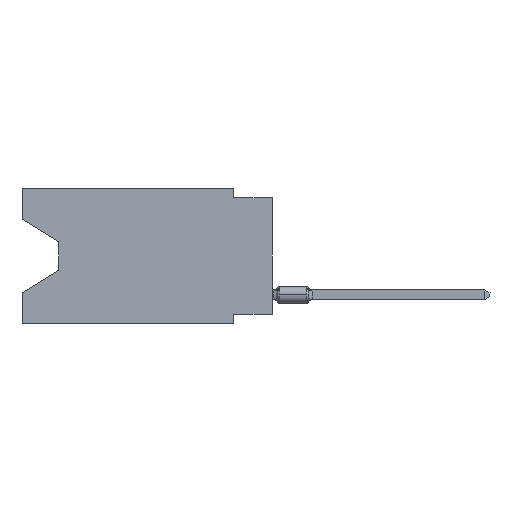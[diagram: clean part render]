
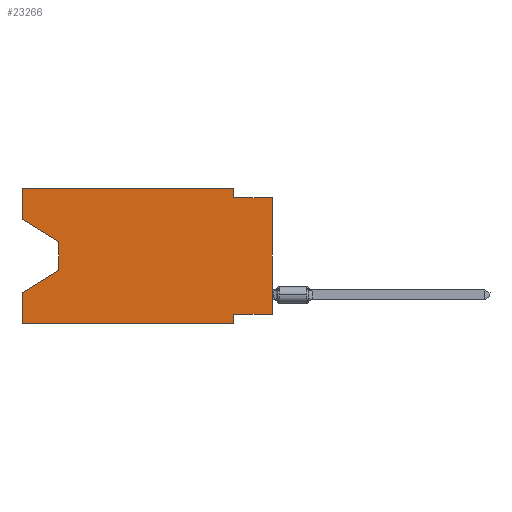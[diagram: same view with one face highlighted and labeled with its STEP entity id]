
A CAD part, left-side view. The second image highlights one B-rep face of the part: STEP entity #23266.
In plain terms, the highlighted planar face has unit normal (-1, 0, 0).
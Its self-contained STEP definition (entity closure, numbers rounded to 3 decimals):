
#442 = EDGE_CURVE ( 'NONE', #22999, #3769, #12356, .T. ) ;
#644 = DIRECTION ( 'NONE',  ( 0., -0.855, -0.519 ) ) ;
#653 = VERTEX_POINT ( 'NONE', #32767 ) ;
#2056 = DIRECTION ( 'NONE',  ( 0., 0., -1. ) ) ;
#2120 = LINE ( 'NONE', #27489, #5346 ) ;
#2389 = VECTOR ( 'NONE', #644, 1000. ) ;
#2647 = CARTESIAN_POINT ( 'NONE',  ( 0., 2.54, 0. ) ) ;
#2671 = EDGE_CURVE ( 'NONE', #15702, #17111, #13819, .T. ) ;
#3279 = DIRECTION ( 'NONE',  ( 0., -1., 0. ) ) ;
#3314 = LINE ( 'NONE', #16324, #17776 ) ;
#3705 = CARTESIAN_POINT ( 'NONE',  ( 0., 16.383, -6.852 ) ) ;
#3769 = VERTEX_POINT ( 'NONE', #3705 ) ;
#4119 = EDGE_CURVE ( 'NONE', #17111, #22999, #9005, .T. ) ;
#5346 = VECTOR ( 'NONE', #17646, 1000. ) ;
#5392 = DIRECTION ( 'NONE',  ( 0., -1., 0. ) ) ;
#5425 = ORIENTED_EDGE ( 'NONE', *, *, #5954, .T. ) ;
#5474 = CARTESIAN_POINT ( 'NONE',  ( 0., 16.383, 0. ) ) ;
#5954 = EDGE_CURVE ( 'NONE', #28334, #21134, #17801, .T. ) ;
#6075 = LINE ( 'NONE', #13913, #18885 ) ;
#6203 = CARTESIAN_POINT ( 'NONE',  ( 0., 13.97, -3.505 ) ) ;
#6635 = ORIENTED_EDGE ( 'NONE', *, *, #13064, .F. ) ;
#7276 = DIRECTION ( 'NONE',  ( 0., 1., 0. ) ) ;
#8796 = VERTEX_POINT ( 'NONE', #28716 ) ;
#9005 = LINE ( 'NONE', #11507, #21116 ) ;
#9385 = VECTOR ( 'NONE', #5392, 1000. ) ;
#9765 = DIRECTION ( 'NONE',  ( 0., -1., 0. ) ) ;
#9788 = ORIENTED_EDGE ( 'NONE', *, *, #12281, .F. ) ;
#9918 = LINE ( 'NONE', #14455, #26642 ) ;
#11176 = CARTESIAN_POINT ( 'NONE',  ( 0., 0., -0.635 ) ) ;
#11317 = DIRECTION ( 'NONE',  ( 0., 0., -1. ) ) ;
#11507 = CARTESIAN_POINT ( 'NONE',  ( 0., 13.97, -3.505 ) ) ;
#12281 = EDGE_CURVE ( 'NONE', #29507, #12724, #3314, .T. ) ;
#12282 = CARTESIAN_POINT ( 'NONE',  ( 0., 2.54, -8.89 ) ) ;
#12356 = LINE ( 'NONE', #27379, #27001 ) ;
#12519 = VECTOR ( 'NONE', #14032, 1000. ) ;
#12667 = ORIENTED_EDGE ( 'NONE', *, *, #13554, .T. ) ;
#12724 = VERTEX_POINT ( 'NONE', #24295 ) ;
#13064 = EDGE_CURVE ( 'NONE', #28334, #3769, #6075, .T. ) ;
#13280 = AXIS2_PLACEMENT_3D ( 'NONE', #20258, #15070, #2056 ) ;
#13554 = EDGE_CURVE ( 'NONE', #8796, #32348, #27857, .T. ) ;
#13819 = LINE ( 'NONE', #23676, #2389 ) ;
#13913 = CARTESIAN_POINT ( 'NONE',  ( 0., 16.383, 0. ) ) ;
#14032 = DIRECTION ( 'NONE',  ( 0., 0., 1. ) ) ;
#14408 = ORIENTED_EDGE ( 'NONE', *, *, #29899, .F. ) ;
#14455 = CARTESIAN_POINT ( 'NONE',  ( 0., 0., -8.255 ) ) ;
#14569 = FACE_OUTER_BOUND ( 'NONE', #31583, .T. ) ;
#14608 = DIRECTION ( 'NONE',  ( 0., 0., -1. ) ) ;
#14662 = CARTESIAN_POINT ( 'NONE',  ( 0., 16.383, 0. ) ) ;
#15070 = DIRECTION ( 'NONE',  ( 1., 0., 0. ) ) ;
#15702 = VERTEX_POINT ( 'NONE', #22621 ) ;
#16131 = ORIENTED_EDGE ( 'NONE', *, *, #31618, .F. ) ;
#16324 = CARTESIAN_POINT ( 'NONE',  ( 0., 2.54, 0. ) ) ;
#17111 = VERTEX_POINT ( 'NONE', #6203 ) ;
#17641 = VERTEX_POINT ( 'NONE', #14662 ) ;
#17646 = DIRECTION ( 'NONE',  ( 0., 0., 1. ) ) ;
#17701 = ORIENTED_EDGE ( 'NONE', *, *, #18612, .F. ) ;
#17754 = EDGE_CURVE ( 'NONE', #12724, #32348, #20912, .T. ) ;
#17776 = VECTOR ( 'NONE', #11317, 1000. ) ;
#17801 = LINE ( 'NONE', #32835, #26101 ) ;
#18319 = LINE ( 'NONE', #5474, #30921 ) ;
#18461 = ORIENTED_EDGE ( 'NONE', *, *, #2671, .T. ) ;
#18612 = EDGE_CURVE ( 'NONE', #653, #21134, #27471, .T. ) ;
#18692 = ORIENTED_EDGE ( 'NONE', *, *, #442, .T. ) ;
#18885 = VECTOR ( 'NONE', #20946, 1000. ) ;
#20258 = CARTESIAN_POINT ( 'NONE',  ( 0., 16.383, 0. ) ) ;
#20323 = ORIENTED_EDGE ( 'NONE', *, *, #24334, .F. ) ;
#20723 = VECTOR ( 'NONE', #14608, 1000. ) ;
#20912 = LINE ( 'NONE', #31421, #9385 ) ;
#20946 = DIRECTION ( 'NONE',  ( 0., 0., 1. ) ) ;
#21116 = VECTOR ( 'NONE', #21535, 1000. ) ;
#21134 = VERTEX_POINT ( 'NONE', #28406 ) ;
#21535 = DIRECTION ( 'NONE',  ( 0., 0., -1. ) ) ;
#22621 = CARTESIAN_POINT ( 'NONE',  ( 0., 16.383, -2.038 ) ) ;
#22999 = VERTEX_POINT ( 'NONE', #25154 ) ;
#23266 = ADVANCED_FACE ( 'NONE', ( #14569 ), #25101, .F. ) ;
#23676 = CARTESIAN_POINT ( 'NONE',  ( 0., 16.383, -2.038 ) ) ;
#24295 = CARTESIAN_POINT ( 'NONE',  ( 0., 2.54, -0.635 ) ) ;
#24334 = EDGE_CURVE ( 'NONE', #15702, #17641, #2120, .T. ) ;
#25014 = CARTESIAN_POINT ( 'NONE',  ( 0., 0., 0. ) ) ;
#25101 = PLANE ( 'NONE',  #13280 ) ;
#25154 = CARTESIAN_POINT ( 'NONE',  ( 0., 13.97, -5.385 ) ) ;
#26101 = VECTOR ( 'NONE', #9765, 1000. ) ;
#26642 = VECTOR ( 'NONE', #7276, 1000. ) ;
#27001 = VECTOR ( 'NONE', #30215, 1000. ) ;
#27379 = CARTESIAN_POINT ( 'NONE',  ( 0., 13.97, -5.385 ) ) ;
#27471 = LINE ( 'NONE', #12282, #20723 ) ;
#27489 = CARTESIAN_POINT ( 'NONE',  ( 0., 16.383, 0. ) ) ;
#27857 = LINE ( 'NONE', #25014, #12519 ) ;
#28334 = VERTEX_POINT ( 'NONE', #32699 ) ;
#28406 = CARTESIAN_POINT ( 'NONE',  ( 0., 2.54, -8.89 ) ) ;
#28716 = CARTESIAN_POINT ( 'NONE',  ( 0., 0., -8.255 ) ) ;
#28934 = ORIENTED_EDGE ( 'NONE', *, *, #4119, .T. ) ;
#29266 = ORIENTED_EDGE ( 'NONE', *, *, #17754, .F. ) ;
#29507 = VERTEX_POINT ( 'NONE', #2647 ) ;
#29899 = EDGE_CURVE ( 'NONE', #8796, #653, #9918, .T. ) ;
#30215 = DIRECTION ( 'NONE',  ( 0., 0.855, -0.519 ) ) ;
#30921 = VECTOR ( 'NONE', #3279, 1000. ) ;
#31421 = CARTESIAN_POINT ( 'NONE',  ( 0., 0., -0.635 ) ) ;
#31583 = EDGE_LOOP ( 'NONE', ( #18461, #28934, #18692, #6635, #5425, #17701, #14408, #12667, #29266, #9788, #16131, #20323 ) ) ;
#31618 = EDGE_CURVE ( 'NONE', #17641, #29507, #18319, .T. ) ;
#32348 = VERTEX_POINT ( 'NONE', #11176 ) ;
#32699 = CARTESIAN_POINT ( 'NONE',  ( 0., 16.383, -8.89 ) ) ;
#32767 = CARTESIAN_POINT ( 'NONE',  ( 0., 2.54, -8.255 ) ) ;
#32835 = CARTESIAN_POINT ( 'NONE',  ( 0., 16.383, -8.89 ) ) ;
